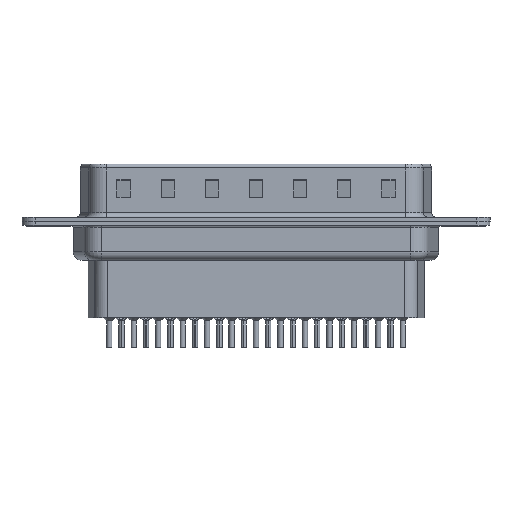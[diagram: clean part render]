
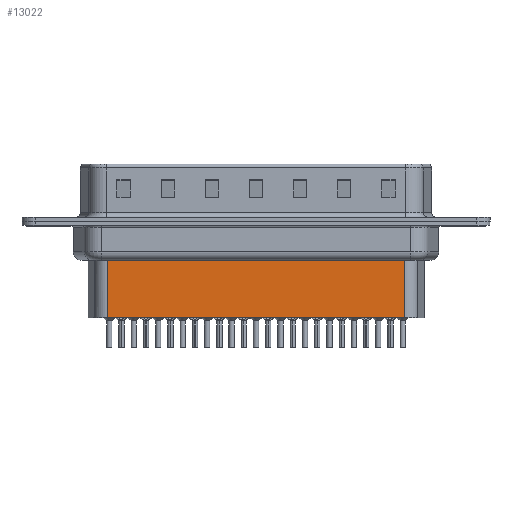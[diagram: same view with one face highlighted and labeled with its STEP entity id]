
A CAD part, front view. The second image highlights one B-rep face of the part: STEP entity #13022.
In plain terms, the highlighted planar face has unit normal (0, -1, 0).
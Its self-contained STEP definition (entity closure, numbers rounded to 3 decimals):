
#320 = LINE ( 'NONE', #10852, #10421 ) ;
#1187 = EDGE_LOOP ( 'NONE', ( #5908, #16037, #3747, #18505 ) ) ;
#2205 = CARTESIAN_POINT ( 'NONE',  ( 6.706, -3.5, -10.95 ) ) ;
#2947 = VECTOR ( 'NONE', #8064, 1000. ) ;
#3154 = VERTEX_POINT ( 'NONE', #20269 ) ;
#3342 = VERTEX_POINT ( 'NONE', #6619 ) ;
#3408 = FACE_OUTER_BOUND ( 'NONE', #1187, .T. ) ;
#3527 = CARTESIAN_POINT ( 'NONE',  ( 6.706, -3.5, -10.95 ) ) ;
#3747 = ORIENTED_EDGE ( 'NONE', *, *, #8090, .T. ) ;
#5346 = VECTOR ( 'NONE', #16438, 1000. ) ;
#5551 = CARTESIAN_POINT ( 'NONE',  ( 6.706, -3.5, -3.1 ) ) ;
#5908 = ORIENTED_EDGE ( 'NONE', *, *, #5931, .F. ) ;
#5931 = EDGE_CURVE ( 'NONE', #17408, #3154, #16194, .T. ) ;
#6619 = CARTESIAN_POINT ( 'NONE',  ( 6.706, -3.5, -4.097 ) ) ;
#6846 = CARTESIAN_POINT ( 'NONE',  ( 40.344, -3.5, -4.097 ) ) ;
#8064 = DIRECTION ( 'NONE',  ( -1., 0., 0. ) ) ;
#8090 = EDGE_CURVE ( 'NONE', #3342, #12996, #320, .T. ) ;
#10421 = VECTOR ( 'NONE', #14700, 1000. ) ;
#10636 = CARTESIAN_POINT ( 'NONE',  ( 6.459, -3.5, -4.097 ) ) ;
#10852 = CARTESIAN_POINT ( 'NONE',  ( 6.706, -3.5, -3.1 ) ) ;
#12996 = VERTEX_POINT ( 'NONE', #3527 ) ;
#13022 = ADVANCED_FACE ( 'NONE', ( #3408 ), #17911, .T. ) ;
#14530 = CARTESIAN_POINT ( 'NONE',  ( 40.344, -3.5, -3.1 ) ) ;
#14700 = DIRECTION ( 'NONE',  ( 0., 0., -1. ) ) ;
#14719 = LINE ( 'NONE', #10636, #2947 ) ;
#16037 = ORIENTED_EDGE ( 'NONE', *, *, #18717, .T. ) ;
#16194 = LINE ( 'NONE', #14530, #5346 ) ;
#16438 = DIRECTION ( 'NONE',  ( 0., 0., -1. ) ) ;
#16736 = AXIS2_PLACEMENT_3D ( 'NONE', #5551, #19813, #18020 ) ;
#17408 = VERTEX_POINT ( 'NONE', #6846 ) ;
#17911 = PLANE ( 'NONE',  #16736 ) ;
#18020 = DIRECTION ( 'NONE',  ( 1., 0., 0. ) ) ;
#18505 = ORIENTED_EDGE ( 'NONE', *, *, #22339, .F. ) ;
#18716 = LINE ( 'NONE', #2205, #18919 ) ;
#18717 = EDGE_CURVE ( 'NONE', #17408, #3342, #14719, .T. ) ;
#18919 = VECTOR ( 'NONE', #22376, 1000. ) ;
#19813 = DIRECTION ( 'NONE',  ( 0., -1., 0. ) ) ;
#20269 = CARTESIAN_POINT ( 'NONE',  ( 40.344, -3.5, -10.95 ) ) ;
#22339 = EDGE_CURVE ( 'NONE', #3154, #12996, #18716, .T. ) ;
#22376 = DIRECTION ( 'NONE',  ( -1., 0., 0. ) ) ;
